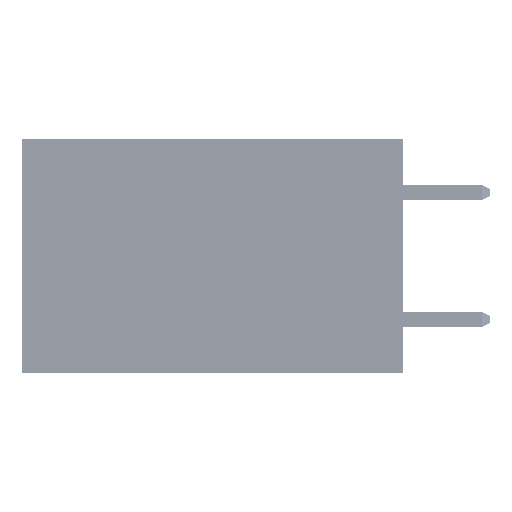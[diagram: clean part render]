
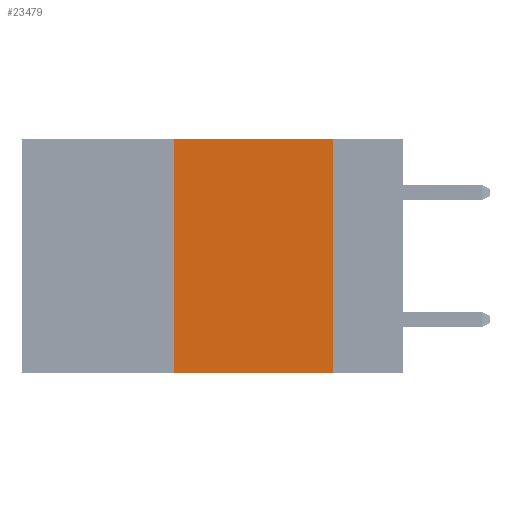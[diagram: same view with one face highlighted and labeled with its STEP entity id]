
A CAD part, left-side view. The second image highlights one B-rep face of the part: STEP entity #23479.
In plain terms, the highlighted planar face has unit normal (-1, 0, 0).
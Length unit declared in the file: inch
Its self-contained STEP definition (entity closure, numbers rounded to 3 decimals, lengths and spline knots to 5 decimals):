
#1655 = VERTEX_POINT ( 'NONE', #45845 ) ;
#3237 = EDGE_CURVE ( 'NONE', #47764, #49570, #14777, .T. ) ;
#5069 = DIRECTION ( 'NONE',  ( 0., 0., -1. ) ) ;
#7233 = LINE ( 'NONE', #49389, #28097 ) ;
#10252 = DIRECTION ( 'NONE',  ( 0., 0., -1. ) ) ;
#10462 = EDGE_CURVE ( 'NONE', #47764, #1655, #13985, .T. ) ;
#11514 = VECTOR ( 'NONE', #50624, 39.37008 ) ;
#11647 = CARTESIAN_POINT ( 'NONE',  ( 0., 0.36, 0. ) ) ;
#13985 = LINE ( 'NONE', #19429, #11514 ) ;
#14777 = LINE ( 'NONE', #11647, #45959 ) ;
#15750 = ORIENTED_EDGE ( 'NONE', *, *, #47851, .F. ) ;
#16210 = VERTEX_POINT ( 'NONE', #25492 ) ;
#19429 = CARTESIAN_POINT ( 'NONE',  ( 0., 0.6, -0.37 ) ) ;
#19789 = CARTESIAN_POINT ( 'NONE',  ( 0., 0.6, 0. ) ) ;
#22500 = CARTESIAN_POINT ( 'NONE',  ( 0., 0.36, 0. ) ) ;
#22512 = ORIENTED_EDGE ( 'NONE', *, *, #10462, .T. ) ;
#23479 = ADVANCED_FACE ( 'NONE', ( #24774 ), #48004, .F. ) ;
#24167 = AXIS2_PLACEMENT_3D ( 'NONE', #24634, #28544, #5069 ) ;
#24634 = CARTESIAN_POINT ( 'NONE',  ( 0., 0.6, 0. ) ) ;
#24774 = FACE_OUTER_BOUND ( 'NONE', #30843, .T. ) ;
#25492 = CARTESIAN_POINT ( 'NONE',  ( 0., 0.11, 0. ) ) ;
#25795 = VECTOR ( 'NONE', #47095, 39.37008 ) ;
#26528 = EDGE_CURVE ( 'NONE', #16210, #1655, #7233, .T. ) ;
#26803 = CARTESIAN_POINT ( 'NONE',  ( 0., 0.36, -0.37 ) ) ;
#28097 = VECTOR ( 'NONE', #10252, 39.37008 ) ;
#28544 = DIRECTION ( 'NONE',  ( 1., 0., 0. ) ) ;
#29423 = ORIENTED_EDGE ( 'NONE', *, *, #26528, .F. ) ;
#30843 = EDGE_LOOP ( 'NONE', ( #29423, #15750, #43254, #22512 ) ) ;
#34929 = LINE ( 'NONE', #19789, #25795 ) ;
#42940 = DIRECTION ( 'NONE',  ( 0., 0., 1. ) ) ;
#43254 = ORIENTED_EDGE ( 'NONE', *, *, #3237, .F. ) ;
#45845 = CARTESIAN_POINT ( 'NONE',  ( 0., 0.11, -0.37 ) ) ;
#45959 = VECTOR ( 'NONE', #42940, 39.37008 ) ;
#47095 = DIRECTION ( 'NONE',  ( 0., -1., 0. ) ) ;
#47764 = VERTEX_POINT ( 'NONE', #26803 ) ;
#47851 = EDGE_CURVE ( 'NONE', #49570, #16210, #34929, .T. ) ;
#48004 = PLANE ( 'NONE',  #24167 ) ;
#49389 = CARTESIAN_POINT ( 'NONE',  ( 0., 0.11, 0. ) ) ;
#49570 = VERTEX_POINT ( 'NONE', #22500 ) ;
#50624 = DIRECTION ( 'NONE',  ( 0., -1., 0. ) ) ;
